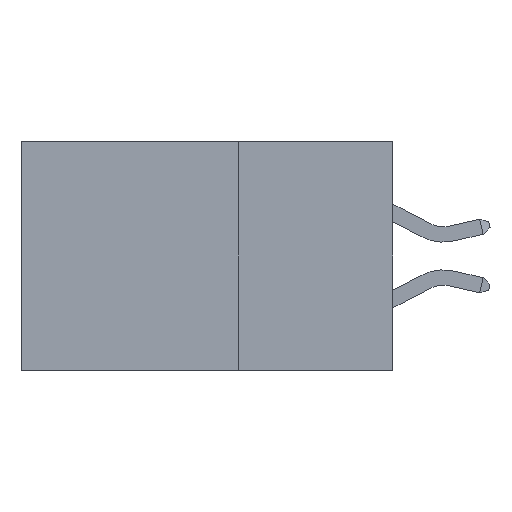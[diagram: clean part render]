
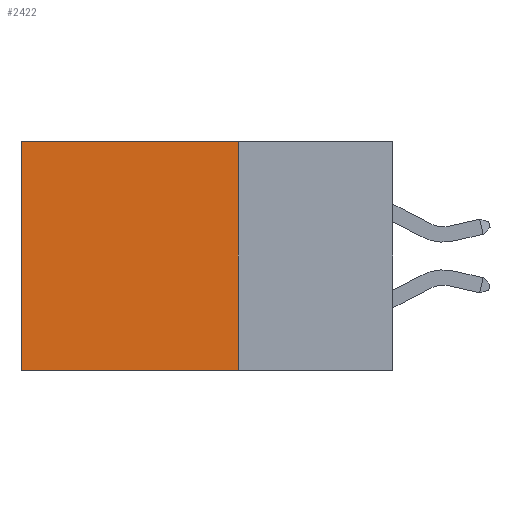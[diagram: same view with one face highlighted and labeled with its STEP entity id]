
A CAD part, left-side view. The second image highlights one B-rep face of the part: STEP entity #2422.
In plain terms, the highlighted planar face has unit normal (-1, 0, 0).
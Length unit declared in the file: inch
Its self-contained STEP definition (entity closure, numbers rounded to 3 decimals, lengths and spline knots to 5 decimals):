
#344 = EDGE_CURVE ( 'NONE', #3637, #4552, #12596, .T. ) ;
#434 = CARTESIAN_POINT ( 'NONE',  ( 0.2875, 0.6, -0.37 ) ) ;
#436 = AXIS2_PLACEMENT_3D ( 'NONE', #3709, #7732, #730 ) ;
#730 = DIRECTION ( 'NONE',  ( 0., 0., -1. ) ) ;
#1603 = VECTOR ( 'NONE', #9546, 39.37008 ) ;
#1682 = LINE ( 'NONE', #2862, #12497 ) ;
#1835 = PLANE ( 'NONE',  #436 ) ;
#1844 = VERTEX_POINT ( 'NONE', #11710 ) ;
#2422 = ADVANCED_FACE ( 'NONE', ( #9611 ), #1835, .F. ) ;
#2471 = DIRECTION ( 'NONE',  ( 0., 1., 0. ) ) ;
#2573 = VECTOR ( 'NONE', #2471, 39.37008 ) ;
#2862 = CARTESIAN_POINT ( 'NONE',  ( 0.2875, 0.25, 0. ) ) ;
#3637 = VERTEX_POINT ( 'NONE', #8283 ) ;
#3709 = CARTESIAN_POINT ( 'NONE',  ( 0.2875, 0.25, 0. ) ) ;
#4202 = EDGE_CURVE ( 'NONE', #4792, #1844, #1682, .T. ) ;
#4545 = CARTESIAN_POINT ( 'NONE',  ( 0.2875, 0.6, 0. ) ) ;
#4552 = VERTEX_POINT ( 'NONE', #434 ) ;
#4781 = DIRECTION ( 'NONE',  ( 0., 0., -1. ) ) ;
#4792 = VERTEX_POINT ( 'NONE', #11846 ) ;
#5419 = LINE ( 'NONE', #10227, #8219 ) ;
#5528 = ORIENTED_EDGE ( 'NONE', *, *, #344, .T. ) ;
#6223 = EDGE_LOOP ( 'NONE', ( #5528, #10295, #11783, #12223 ) ) ;
#7519 = CARTESIAN_POINT ( 'NONE',  ( 0.2875, 0.25, -0.37 ) ) ;
#7602 = EDGE_CURVE ( 'NONE', #4792, #3637, #5419, .T. ) ;
#7732 = DIRECTION ( 'NONE',  ( 1., 0., 0. ) ) ;
#8219 = VECTOR ( 'NONE', #10162, 39.37008 ) ;
#8283 = CARTESIAN_POINT ( 'NONE',  ( 0.2875, 0.6, 0. ) ) ;
#9546 = DIRECTION ( 'NONE',  ( 0., 0., -1. ) ) ;
#9611 = FACE_OUTER_BOUND ( 'NONE', #6223, .T. ) ;
#10162 = DIRECTION ( 'NONE',  ( 0., 1., 0. ) ) ;
#10227 = CARTESIAN_POINT ( 'NONE',  ( 0.2875, 0.25, 0. ) ) ;
#10295 = ORIENTED_EDGE ( 'NONE', *, *, #12459, .F. ) ;
#10523 = LINE ( 'NONE', #7519, #2573 ) ;
#11710 = CARTESIAN_POINT ( 'NONE',  ( 0.2875, 0.25, -0.37 ) ) ;
#11783 = ORIENTED_EDGE ( 'NONE', *, *, #4202, .F. ) ;
#11846 = CARTESIAN_POINT ( 'NONE',  ( 0.2875, 0.25, 0. ) ) ;
#12223 = ORIENTED_EDGE ( 'NONE', *, *, #7602, .T. ) ;
#12459 = EDGE_CURVE ( 'NONE', #1844, #4552, #10523, .T. ) ;
#12497 = VECTOR ( 'NONE', #4781, 39.37008 ) ;
#12596 = LINE ( 'NONE', #4545, #1603 ) ;
